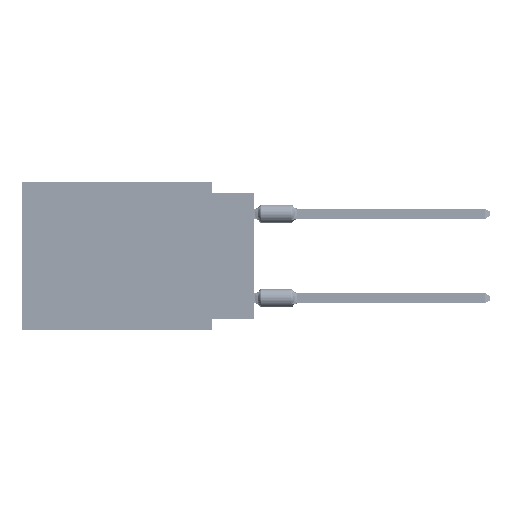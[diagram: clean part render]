
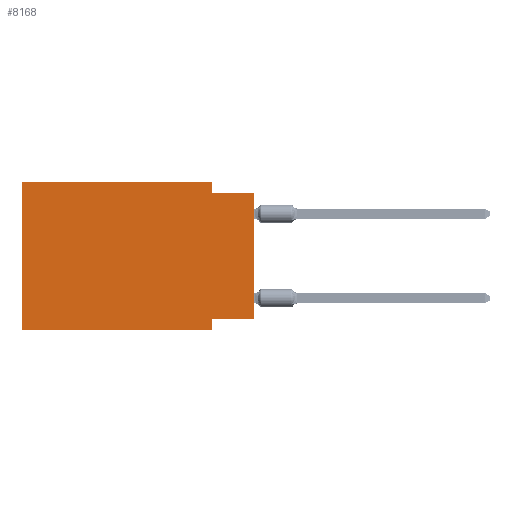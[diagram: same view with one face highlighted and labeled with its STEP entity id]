
A CAD part, left-side view. The second image highlights one B-rep face of the part: STEP entity #8168.
In plain terms, the highlighted planar face has unit normal (-1, 0, 0).
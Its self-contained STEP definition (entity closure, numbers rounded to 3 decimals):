
#865 = CARTESIAN_POINT ( 'NONE',  ( 0., 2.54, 0. ) ) ;
#2611 = DIRECTION ( 'NONE',  ( 0., 0., -1. ) ) ;
#3921 = VERTEX_POINT ( 'NONE', #26586 ) ;
#4211 = LINE ( 'NONE', #65007, #11810 ) ;
#5497 = EDGE_LOOP ( 'NONE', ( #51465, #51035, #16993, #76198, #25261, #8529, #63327, #33656 ) ) ;
#8168 = ADVANCED_FACE ( 'NONE', ( #89711 ), #76219, .F. ) ;
#8529 = ORIENTED_EDGE ( 'NONE', *, *, #36734, .T. ) ;
#10152 = LINE ( 'NONE', #63956, #52005 ) ;
#11810 = VECTOR ( 'NONE', #95410, 1000. ) ;
#13195 = VECTOR ( 'NONE', #2611, 1000. ) ;
#14268 = CARTESIAN_POINT ( 'NONE',  ( 0., 0., -0.635 ) ) ;
#16993 = ORIENTED_EDGE ( 'NONE', *, *, #25729, .F. ) ;
#17443 = CARTESIAN_POINT ( 'NONE',  ( 0., 0., 0. ) ) ;
#18363 = VECTOR ( 'NONE', #63128, 1000. ) ;
#21413 = CARTESIAN_POINT ( 'NONE',  ( 0., 13.97, 0. ) ) ;
#21486 = VERTEX_POINT ( 'NONE', #65917 ) ;
#23496 = CARTESIAN_POINT ( 'NONE',  ( 0., 0., -8.255 ) ) ;
#24052 = CARTESIAN_POINT ( 'NONE',  ( 0., 2.54, -8.255 ) ) ;
#25261 = ORIENTED_EDGE ( 'NONE', *, *, #97405, .F. ) ;
#25729 = EDGE_CURVE ( 'NONE', #3921, #77275, #38249, .T. ) ;
#26586 = CARTESIAN_POINT ( 'NONE',  ( 0., 2.54, 0. ) ) ;
#28660 = EDGE_CURVE ( 'NONE', #42772, #85060, #49800, .T. ) ;
#28918 = CARTESIAN_POINT ( 'NONE',  ( 0., 13.97, 0. ) ) ;
#30019 = VERTEX_POINT ( 'NONE', #65725 ) ;
#32397 = DIRECTION ( 'NONE',  ( 0., 0., 1. ) ) ;
#33397 = VECTOR ( 'NONE', #70275, 1000. ) ;
#33656 = ORIENTED_EDGE ( 'NONE', *, *, #75996, .F. ) ;
#33995 = LINE ( 'NONE', #78839, #13195 ) ;
#34931 = LINE ( 'NONE', #28918, #54556 ) ;
#36734 = EDGE_CURVE ( 'NONE', #84697, #21486, #64267, .T. ) ;
#38249 = LINE ( 'NONE', #865, #18363 ) ;
#40523 = VECTOR ( 'NONE', #32397, 1000. ) ;
#42772 = VERTEX_POINT ( 'NONE', #23496 ) ;
#44194 = VECTOR ( 'NONE', #49853, 1000. ) ;
#45063 = AXIS2_PLACEMENT_3D ( 'NONE', #21413, #61268, #52817 ) ;
#47653 = EDGE_CURVE ( 'NONE', #77275, #85060, #97172, .T. ) ;
#49800 = LINE ( 'NONE', #17443, #40523 ) ;
#49853 = DIRECTION ( 'NONE',  ( 0., -1., 0. ) ) ;
#51035 = ORIENTED_EDGE ( 'NONE', *, *, #47653, .F. ) ;
#51465 = ORIENTED_EDGE ( 'NONE', *, *, #28660, .T. ) ;
#52005 = VECTOR ( 'NONE', #55987, 1000. ) ;
#52817 = DIRECTION ( 'NONE',  ( 0., 0., -1. ) ) ;
#54556 = VECTOR ( 'NONE', #83218, 1000. ) ;
#55808 = CARTESIAN_POINT ( 'NONE',  ( 0., 13.97, -8.89 ) ) ;
#55987 = DIRECTION ( 'NONE',  ( 0., 1., 0. ) ) ;
#57322 = CARTESIAN_POINT ( 'NONE',  ( 0., 0., -0.635 ) ) ;
#61268 = DIRECTION ( 'NONE',  ( 1., 0., 0. ) ) ;
#63128 = DIRECTION ( 'NONE',  ( 0., 0., -1. ) ) ;
#63327 = ORIENTED_EDGE ( 'NONE', *, *, #83901, .F. ) ;
#63956 = CARTESIAN_POINT ( 'NONE',  ( 0., 0., -8.255 ) ) ;
#64267 = LINE ( 'NONE', #55808, #33397 ) ;
#65007 = CARTESIAN_POINT ( 'NONE',  ( 0., 13.97, 0. ) ) ;
#65725 = CARTESIAN_POINT ( 'NONE',  ( 0., 13.97, 0. ) ) ;
#65917 = CARTESIAN_POINT ( 'NONE',  ( 0., 2.54, -8.89 ) ) ;
#66920 = CARTESIAN_POINT ( 'NONE',  ( 0., 2.54, -0.635 ) ) ;
#67235 = EDGE_CURVE ( 'NONE', #30019, #3921, #34931, .T. ) ;
#67707 = CARTESIAN_POINT ( 'NONE',  ( 0., 13.97, -8.89 ) ) ;
#70275 = DIRECTION ( 'NONE',  ( 0., -1., 0. ) ) ;
#75996 = EDGE_CURVE ( 'NONE', #42772, #90817, #10152, .T. ) ;
#76198 = ORIENTED_EDGE ( 'NONE', *, *, #67235, .F. ) ;
#76219 = PLANE ( 'NONE',  #45063 ) ;
#77275 = VERTEX_POINT ( 'NONE', #66920 ) ;
#78839 = CARTESIAN_POINT ( 'NONE',  ( 0., 2.54, -8.89 ) ) ;
#83218 = DIRECTION ( 'NONE',  ( 0., -1., 0. ) ) ;
#83901 = EDGE_CURVE ( 'NONE', #90817, #21486, #33995, .T. ) ;
#84697 = VERTEX_POINT ( 'NONE', #67707 ) ;
#85060 = VERTEX_POINT ( 'NONE', #14268 ) ;
#89711 = FACE_OUTER_BOUND ( 'NONE', #5497, .T. ) ;
#90817 = VERTEX_POINT ( 'NONE', #24052 ) ;
#95410 = DIRECTION ( 'NONE',  ( 0., 0., 1. ) ) ;
#97172 = LINE ( 'NONE', #57322, #44194 ) ;
#97405 = EDGE_CURVE ( 'NONE', #84697, #30019, #4211, .T. ) ;
